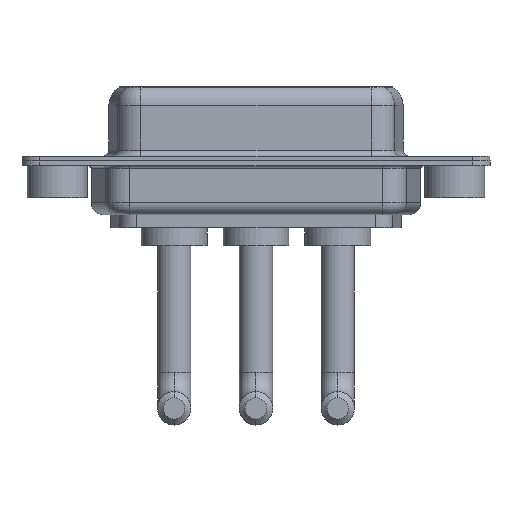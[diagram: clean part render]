
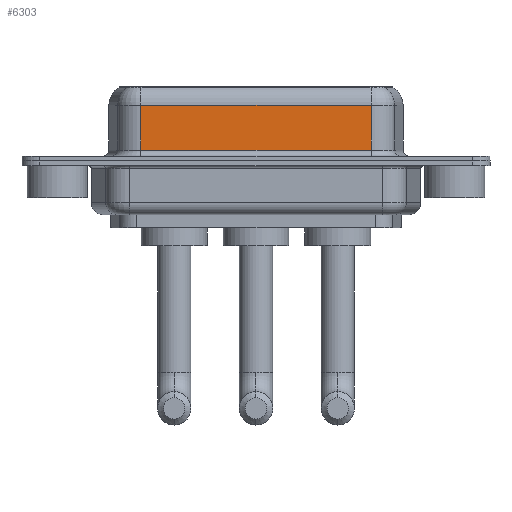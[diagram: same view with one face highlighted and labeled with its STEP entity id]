
A CAD part, front view. The second image highlights one B-rep face of the part: STEP entity #6303.
In plain terms, the highlighted planar face has unit normal (0, -1, 0).
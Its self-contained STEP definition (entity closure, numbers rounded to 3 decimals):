
#164 = ORIENTED_EDGE ( 'NONE', *, *, #2525, .T. ) ;
#1163 = CARTESIAN_POINT ( 'NONE',  ( 26.287, -3.95, 0.9 ) ) ;
#1246 = AXIS2_PLACEMENT_3D ( 'NONE', #8086, #9860, #11922 ) ;
#1606 = EDGE_LOOP ( 'NONE', ( #8051, #11640, #164, #3001 ) ) ;
#1687 = PLANE ( 'NONE',  #1246 ) ;
#1747 = VERTEX_POINT ( 'NONE', #2535 ) ;
#2248 = DIRECTION ( 'NONE',  ( 1., 0., 0. ) ) ;
#2332 = CARTESIAN_POINT ( 'NONE',  ( 7.013, -3.95, 4.65 ) ) ;
#2525 = EDGE_CURVE ( 'NONE', #3397, #9152, #11067, .T. ) ;
#2535 = CARTESIAN_POINT ( 'NONE',  ( 26.287, -3.95, 4.65 ) ) ;
#3001 = ORIENTED_EDGE ( 'NONE', *, *, #9831, .T. ) ;
#3397 = VERTEX_POINT ( 'NONE', #2332 ) ;
#3613 = VECTOR ( 'NONE', #9235, 1000. ) ;
#3747 = LINE ( 'NONE', #11447, #5260 ) ;
#3833 = LINE ( 'NONE', #7635, #9749 ) ;
#5260 = VECTOR ( 'NONE', #10323, 1000. ) ;
#5452 = EDGE_CURVE ( 'NONE', #1747, #8657, #3747, .T. ) ;
#5901 = DIRECTION ( 'NONE',  ( -1., 0., 0. ) ) ;
#6303 = ADVANCED_FACE ( 'NONE', ( #6451 ), #1687, .F. ) ;
#6451 = FACE_OUTER_BOUND ( 'NONE', #1606, .T. ) ;
#7635 = CARTESIAN_POINT ( 'NONE',  ( 26.287, -3.95, 4.65 ) ) ;
#7873 = LINE ( 'NONE', #8936, #11909 ) ;
#8051 = ORIENTED_EDGE ( 'NONE', *, *, #5452, .F. ) ;
#8086 = CARTESIAN_POINT ( 'NONE',  ( 26.287, -3.95, 6.4 ) ) ;
#8657 = VERTEX_POINT ( 'NONE', #1163 ) ;
#8936 = CARTESIAN_POINT ( 'NONE',  ( 26.287, -3.95, 0.9 ) ) ;
#9152 = VERTEX_POINT ( 'NONE', #10342 ) ;
#9235 = DIRECTION ( 'NONE',  ( 0., 0., -1. ) ) ;
#9749 = VECTOR ( 'NONE', #5901, 1000. ) ;
#9831 = EDGE_CURVE ( 'NONE', #9152, #8657, #7873, .T. ) ;
#9860 = DIRECTION ( 'NONE',  ( 0., 1., 0. ) ) ;
#10002 = CARTESIAN_POINT ( 'NONE',  ( 7.013, -3.95, 6.4 ) ) ;
#10323 = DIRECTION ( 'NONE',  ( 0., 0., -1. ) ) ;
#10342 = CARTESIAN_POINT ( 'NONE',  ( 7.013, -3.95, 0.9 ) ) ;
#11067 = LINE ( 'NONE', #10002, #3613 ) ;
#11210 = EDGE_CURVE ( 'NONE', #1747, #3397, #3833, .T. ) ;
#11447 = CARTESIAN_POINT ( 'NONE',  ( 26.287, -3.95, 6.4 ) ) ;
#11640 = ORIENTED_EDGE ( 'NONE', *, *, #11210, .T. ) ;
#11909 = VECTOR ( 'NONE', #2248, 1000. ) ;
#11922 = DIRECTION ( 'NONE',  ( 0., 0., 1. ) ) ;
